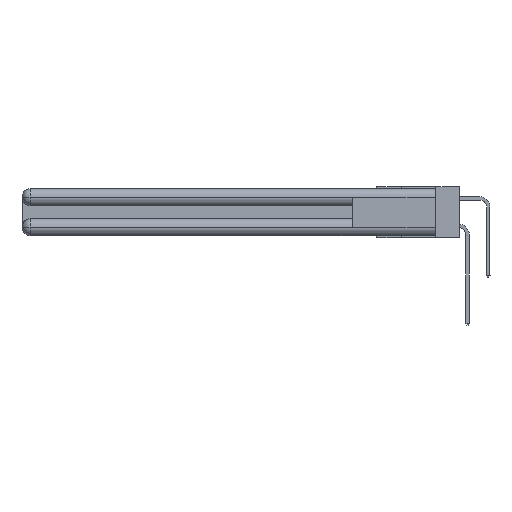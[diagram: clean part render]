
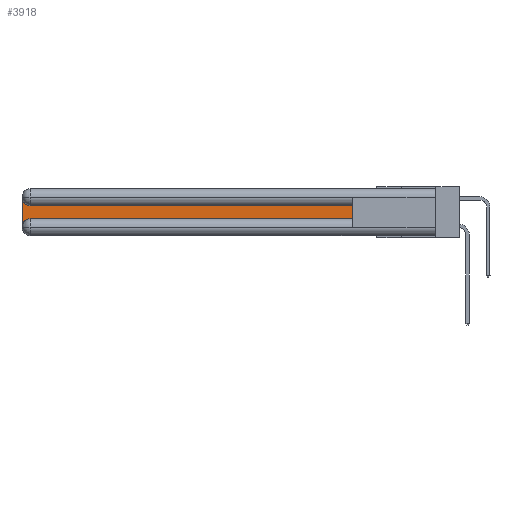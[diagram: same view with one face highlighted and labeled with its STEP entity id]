
A CAD part, left-side view. The second image highlights one B-rep face of the part: STEP entity #3918.
In plain terms, the highlighted planar face has unit normal (-1, 0, 0).
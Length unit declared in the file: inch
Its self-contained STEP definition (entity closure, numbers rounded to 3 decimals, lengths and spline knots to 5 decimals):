
#85 = ORIENTED_EDGE ( 'NONE', *, *, #9547, .T. ) ;
#190 = ORIENTED_EDGE ( 'NONE', *, *, #3202, .T. ) ;
#316 = FACE_OUTER_BOUND ( 'NONE', #22047, .T. ) ;
#2036 = LINE ( 'NONE', #9952, #16548 ) ;
#2448 = CARTESIAN_POINT ( 'NONE',  ( 0.075, 3., -0.2175 ) ) ;
#2612 = CARTESIAN_POINT ( 'NONE',  ( 0.075, 3., -0.1225 ) ) ;
#3111 = CARTESIAN_POINT ( 'NONE',  ( 0.075, 3., -0.2775 ) ) ;
#3202 = EDGE_CURVE ( 'NONE', #12277, #30177, #3543, .T. ) ;
#3543 = LINE ( 'NONE', #2448, #16105 ) ;
#3918 = ADVANCED_FACE ( 'NONE', ( #316 ), #32444, .F. ) ;
#3989 = ORIENTED_EDGE ( 'NONE', *, *, #28883, .T. ) ;
#6328 = DIRECTION ( 'NONE',  ( 0., 0., -1. ) ) ;
#6850 = CARTESIAN_POINT ( 'NONE',  ( 0.075, 3., -0.0625 ) ) ;
#7458 = AXIS2_PLACEMENT_3D ( 'NONE', #2612, #22607, #22720 ) ;
#7494 = VERTEX_POINT ( 'NONE', #16116 ) ;
#7977 = CARTESIAN_POINT ( 'NONE',  ( 0.075, 0.6, -0.2175 ) ) ;
#8793 = CARTESIAN_POINT ( 'NONE',  ( 0.075, 0.6, -0.2175 ) ) ;
#9547 = EDGE_CURVE ( 'NONE', #30177, #24603, #20580, .T. ) ;
#9897 = LINE ( 'NONE', #12315, #27664 ) ;
#9939 = CIRCLE ( 'NONE', #23765, 0.06 ) ;
#9952 = CARTESIAN_POINT ( 'NONE',  ( 0.075, 0.6, -0.1225 ) ) ;
#12157 = AXIS2_PLACEMENT_3D ( 'NONE', #31858, #29458, #6328 ) ;
#12277 = VERTEX_POINT ( 'NONE', #6850 ) ;
#12315 = CARTESIAN_POINT ( 'NONE',  ( 0.075, 0.6, -0.2175 ) ) ;
#14235 = VERTEX_POINT ( 'NONE', #8793 ) ;
#14600 = DIRECTION ( 'NONE',  ( 0., 0., 1. ) ) ;
#15060 = EDGE_CURVE ( 'NONE', #15702, #7494, #2036, .T. ) ;
#15702 = VERTEX_POINT ( 'NONE', #17028 ) ;
#15754 = CARTESIAN_POINT ( 'NONE',  ( 0.075, 2.94, -0.0625 ) ) ;
#16105 = VECTOR ( 'NONE', #22539, 39.37008 ) ;
#16116 = CARTESIAN_POINT ( 'NONE',  ( 0.075, 2.94, -0.1225 ) ) ;
#16548 = VECTOR ( 'NONE', #27720, 39.37008 ) ;
#17028 = CARTESIAN_POINT ( 'NONE',  ( 0.075, 0.6, -0.1225 ) ) ;
#18085 = DIRECTION ( 'NONE',  ( 0., -1., 0. ) ) ;
#19598 = VECTOR ( 'NONE', #18085, 39.37008 ) ;
#20580 = CIRCLE ( 'NONE', #12157, 0.06 ) ;
#20754 = ORIENTED_EDGE ( 'NONE', *, *, #24969, .T. ) ;
#20782 = LINE ( 'NONE', #7977, #19598 ) ;
#22038 = ORIENTED_EDGE ( 'NONE', *, *, #23085, .T. ) ;
#22047 = EDGE_LOOP ( 'NONE', ( #24518, #3989, #190, #85, #20754, #22038 ) ) ;
#22539 = DIRECTION ( 'NONE',  ( 0., 0., -1. ) ) ;
#22607 = DIRECTION ( 'NONE',  ( 1., 0., 0. ) ) ;
#22720 = DIRECTION ( 'NONE',  ( 0., 0., -1. ) ) ;
#22848 = CARTESIAN_POINT ( 'NONE',  ( 0.075, 2.94, -0.2175 ) ) ;
#23085 = EDGE_CURVE ( 'NONE', #14235, #15702, #9897, .T. ) ;
#23765 = AXIS2_PLACEMENT_3D ( 'NONE', #15754, #31113, #28573 ) ;
#24518 = ORIENTED_EDGE ( 'NONE', *, *, #15060, .T. ) ;
#24603 = VERTEX_POINT ( 'NONE', #22848 ) ;
#24969 = EDGE_CURVE ( 'NONE', #24603, #14235, #20782, .T. ) ;
#27664 = VECTOR ( 'NONE', #14600, 39.37008 ) ;
#27720 = DIRECTION ( 'NONE',  ( 0., 1., 0. ) ) ;
#28573 = DIRECTION ( 'NONE',  ( 0., 0., -1. ) ) ;
#28883 = EDGE_CURVE ( 'NONE', #7494, #12277, #9939, .T. ) ;
#29458 = DIRECTION ( 'NONE',  ( 1., 0., 0. ) ) ;
#30177 = VERTEX_POINT ( 'NONE', #3111 ) ;
#31113 = DIRECTION ( 'NONE',  ( 1., 0., 0. ) ) ;
#31858 = CARTESIAN_POINT ( 'NONE',  ( 0.075, 2.94, -0.2775 ) ) ;
#32444 = PLANE ( 'NONE',  #7458 ) ;
